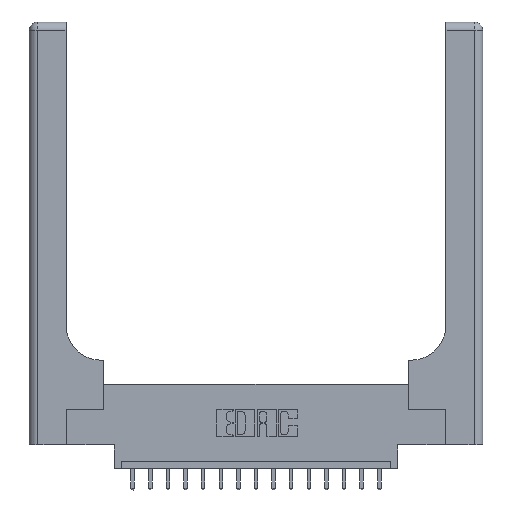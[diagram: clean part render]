
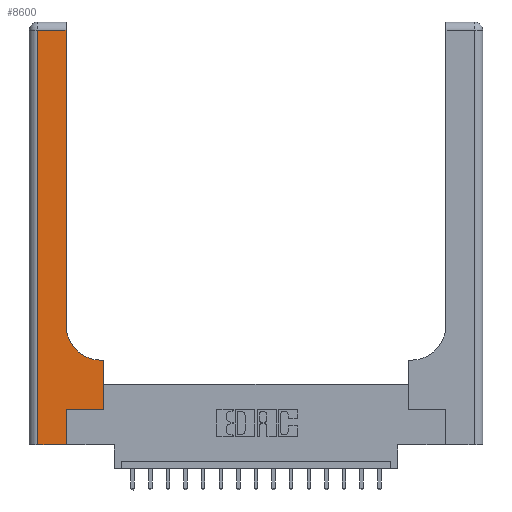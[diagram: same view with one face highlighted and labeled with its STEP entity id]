
A CAD part, top view. The second image highlights one B-rep face of the part: STEP entity #8600.
In plain terms, the highlighted planar face has unit normal (0, 0, 1).
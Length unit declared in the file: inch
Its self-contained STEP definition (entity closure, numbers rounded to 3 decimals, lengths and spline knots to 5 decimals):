
#93 = CARTESIAN_POINT ( 'NONE',  ( 0.26, 0.85, 0.37 ) ) ;
#144 = ORIENTED_EDGE ( 'NONE', *, *, #7790, .T. ) ;
#204 = CARTESIAN_POINT ( 'NONE',  ( 0., 2.94, 0.37 ) ) ;
#286 = CARTESIAN_POINT ( 'NONE',  ( 0.06, 0., 0.37 ) ) ;
#296 = EDGE_CURVE ( 'NONE', #15180, #2319, #8188, .T. ) ;
#369 = VERTEX_POINT ( 'NONE', #14838 ) ;
#611 = EDGE_CURVE ( 'NONE', #2996, #4183, #14562, .T. ) ;
#708 = EDGE_CURVE ( 'NONE', #8308, #15180, #4257, .T. ) ;
#724 = DIRECTION ( 'NONE',  ( 1., 0., 0. ) ) ;
#1080 = LINE ( 'NONE', #5426, #8141 ) ;
#1346 = VECTOR ( 'NONE', #17045, 39.37008 ) ;
#1496 = LINE ( 'NONE', #6764, #16236 ) ;
#1814 = EDGE_CURVE ( 'NONE', #7991, #2996, #1080, .T. ) ;
#1868 = CARTESIAN_POINT ( 'NONE',  ( 0.26, 2.94, 0.37 ) ) ;
#2319 = VERTEX_POINT ( 'NONE', #93 ) ;
#2378 = VECTOR ( 'NONE', #5523, 39.37008 ) ;
#2436 = ORIENTED_EDGE ( 'NONE', *, *, #11320, .T. ) ;
#2816 = FACE_OUTER_BOUND ( 'NONE', #17707, .T. ) ;
#2996 = VERTEX_POINT ( 'NONE', #10514 ) ;
#3540 = PLANE ( 'NONE',  #14569 ) ;
#3590 = ORIENTED_EDGE ( 'NONE', *, *, #611, .T. ) ;
#3920 = CARTESIAN_POINT ( 'NONE',  ( 0.265, 0.25, 0.37 ) ) ;
#3990 = CARTESIAN_POINT ( 'NONE',  ( 0.265, 0., 0.37 ) ) ;
#4183 = VERTEX_POINT ( 'NONE', #3920 ) ;
#4257 = LINE ( 'NONE', #17103, #1346 ) ;
#4392 = CARTESIAN_POINT ( 'NONE',  ( 0.26, 3., 0.37 ) ) ;
#4633 = AXIS2_PLACEMENT_3D ( 'NONE', #11763, #7696, #724 ) ;
#5024 = CARTESIAN_POINT ( 'NONE',  ( 0., 3., 0.37 ) ) ;
#5030 = ORIENTED_EDGE ( 'NONE', *, *, #296, .T. ) ;
#5426 = CARTESIAN_POINT ( 'NONE',  ( 0., 0., 0.37 ) ) ;
#5523 = DIRECTION ( 'NONE',  ( 1., 0., 0. ) ) ;
#6053 = LINE ( 'NONE', #4392, #7352 ) ;
#6642 = VECTOR ( 'NONE', #9776, 39.37008 ) ;
#6764 = CARTESIAN_POINT ( 'NONE',  ( 0.528, 0.25, 0.37 ) ) ;
#7064 = DIRECTION ( 'NONE',  ( 1., 0., 0. ) ) ;
#7100 = CARTESIAN_POINT ( 'NONE',  ( 0.06, 3., 0.37 ) ) ;
#7221 = DIRECTION ( 'NONE',  ( 0., -1., 0. ) ) ;
#7251 = ORIENTED_EDGE ( 'NONE', *, *, #15218, .T. ) ;
#7352 = VECTOR ( 'NONE', #12852, 39.37008 ) ;
#7696 = DIRECTION ( 'NONE',  ( 0., 0., -1. ) ) ;
#7790 = EDGE_CURVE ( 'NONE', #9053, #8308, #1496, .T. ) ;
#7991 = VERTEX_POINT ( 'NONE', #286 ) ;
#8141 = VECTOR ( 'NONE', #7064, 39.37008 ) ;
#8188 = CIRCLE ( 'NONE', #4633, 0.25 ) ;
#8308 = VERTEX_POINT ( 'NONE', #12586 ) ;
#8320 = EDGE_CURVE ( 'NONE', #369, #7991, #14463, .T. ) ;
#8403 = LINE ( 'NONE', #204, #16534 ) ;
#8600 = ADVANCED_FACE ( 'NONE', ( #2816 ), #3540, .F. ) ;
#9053 = VERTEX_POINT ( 'NONE', #13228 ) ;
#9400 = ORIENTED_EDGE ( 'NONE', *, *, #18226, .T. ) ;
#9407 = LINE ( 'NONE', #13924, #2378 ) ;
#9644 = DIRECTION ( 'NONE',  ( 0., 1., 0. ) ) ;
#9776 = DIRECTION ( 'NONE',  ( 0., 1., 0. ) ) ;
#10227 = DIRECTION ( 'NONE',  ( -1., 0., 0. ) ) ;
#10514 = CARTESIAN_POINT ( 'NONE',  ( 0.265, 0., 0.37 ) ) ;
#11320 = EDGE_CURVE ( 'NONE', #2319, #14720, #6053, .T. ) ;
#11763 = CARTESIAN_POINT ( 'NONE',  ( 0.51, 0.85, 0.37 ) ) ;
#12586 = CARTESIAN_POINT ( 'NONE',  ( 0.528, 0.6, 0.37 ) ) ;
#12852 = DIRECTION ( 'NONE',  ( 0., 1., 0. ) ) ;
#13228 = CARTESIAN_POINT ( 'NONE',  ( 0.528, 0.25, 0.37 ) ) ;
#13924 = CARTESIAN_POINT ( 'NONE',  ( 0.265, 0.25, 0.37 ) ) ;
#14170 = CARTESIAN_POINT ( 'NONE',  ( 0.51, 0.6, 0.37 ) ) ;
#14463 = LINE ( 'NONE', #7100, #17777 ) ;
#14483 = ORIENTED_EDGE ( 'NONE', *, *, #708, .T. ) ;
#14562 = LINE ( 'NONE', #3990, #6642 ) ;
#14569 = AXIS2_PLACEMENT_3D ( 'NONE', #5024, #16554, #17988 ) ;
#14720 = VERTEX_POINT ( 'NONE', #1868 ) ;
#14838 = CARTESIAN_POINT ( 'NONE',  ( 0.06, 2.94, 0.37 ) ) ;
#15180 = VERTEX_POINT ( 'NONE', #14170 ) ;
#15218 = EDGE_CURVE ( 'NONE', #4183, #9053, #9407, .T. ) ;
#15975 = ORIENTED_EDGE ( 'NONE', *, *, #1814, .T. ) ;
#16236 = VECTOR ( 'NONE', #9644, 39.37008 ) ;
#16534 = VECTOR ( 'NONE', #10227, 39.37008 ) ;
#16554 = DIRECTION ( 'NONE',  ( 0., 0., -1. ) ) ;
#17045 = DIRECTION ( 'NONE',  ( -1., 0., 0. ) ) ;
#17103 = CARTESIAN_POINT ( 'NONE',  ( 0.26, 0.6, 0.37 ) ) ;
#17173 = ORIENTED_EDGE ( 'NONE', *, *, #8320, .T. ) ;
#17707 = EDGE_LOOP ( 'NONE', ( #2436, #9400, #17173, #15975, #3590, #7251, #144, #14483, #5030 ) ) ;
#17777 = VECTOR ( 'NONE', #7221, 39.37008 ) ;
#17988 = DIRECTION ( 'NONE',  ( -1., 0., 0. ) ) ;
#18226 = EDGE_CURVE ( 'NONE', #14720, #369, #8403, .T. ) ;
